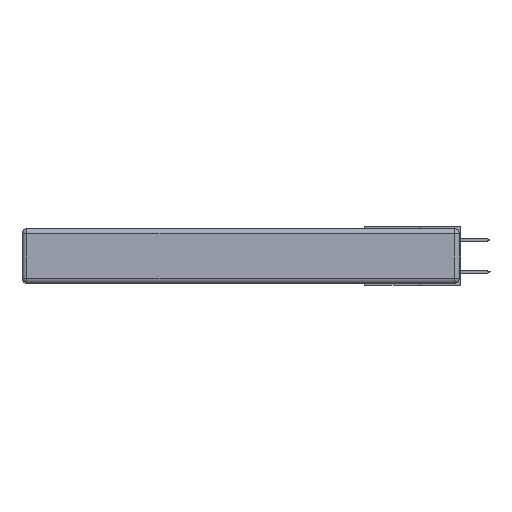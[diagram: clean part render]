
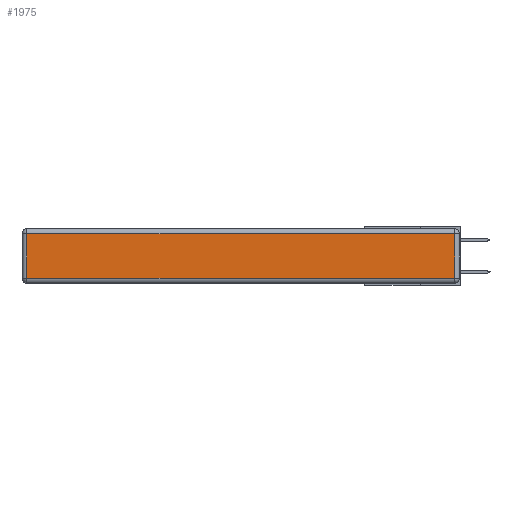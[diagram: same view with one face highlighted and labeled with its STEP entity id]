
A CAD part, left-side view. The second image highlights one B-rep face of the part: STEP entity #1975.
In plain terms, the highlighted planar face has unit normal (-1, 0, 0).
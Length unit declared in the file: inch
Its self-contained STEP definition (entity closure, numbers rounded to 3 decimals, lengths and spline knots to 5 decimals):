
#149 = LINE ( 'NONE', #11013, #15096 ) ;
#1152 = EDGE_CURVE ( 'NONE', #13067, #14570, #5375, .T. ) ;
#1941 = DIRECTION ( 'NONE',  ( 0., 0., -1. ) ) ;
#1975 = ADVANCED_FACE ( 'NONE', ( #10349 ), #14924, .T. ) ;
#2583 = VECTOR ( 'NONE', #1941, 39.37008 ) ;
#2803 = DIRECTION ( 'NONE',  ( 0., 0., 1. ) ) ;
#2914 = CARTESIAN_POINT ( 'NONE',  ( 0., 0.03, -0.03 ) ) ;
#4265 = ORIENTED_EDGE ( 'NONE', *, *, #11725, .T. ) ;
#4637 = VECTOR ( 'NONE', #11472, 39.37008 ) ;
#4708 = ORIENTED_EDGE ( 'NONE', *, *, #6170, .T. ) ;
#5375 = LINE ( 'NONE', #6583, #4637 ) ;
#5457 = EDGE_LOOP ( 'NONE', ( #12188, #4265, #4708, #12010 ) ) ;
#6170 = EDGE_CURVE ( 'NONE', #7872, #12443, #10819, .T. ) ;
#6190 = AXIS2_PLACEMENT_3D ( 'NONE', #7785, #9056, #9099 ) ;
#6583 = CARTESIAN_POINT ( 'NONE',  ( 0., 0., -0.313 ) ) ;
#7785 = CARTESIAN_POINT ( 'NONE',  ( 0., 0., -0.343 ) ) ;
#7872 = VERTEX_POINT ( 'NONE', #2914 ) ;
#7988 = DIRECTION ( 'NONE',  ( 0., 1., 0. ) ) ;
#8191 = VECTOR ( 'NONE', #7988, 39.37008 ) ;
#8332 = CARTESIAN_POINT ( 'NONE',  ( 0., 2.72, -0.313 ) ) ;
#9056 = DIRECTION ( 'NONE',  ( -1., 0., 0. ) ) ;
#9099 = DIRECTION ( 'NONE',  ( 0., 0., 1. ) ) ;
#10349 = FACE_OUTER_BOUND ( 'NONE', #5457, .T. ) ;
#10819 = LINE ( 'NONE', #11369, #8191 ) ;
#11013 = CARTESIAN_POINT ( 'NONE',  ( 0., 0.03, -0.343 ) ) ;
#11369 = CARTESIAN_POINT ( 'NONE',  ( 0., 2.75, -0.03 ) ) ;
#11404 = CARTESIAN_POINT ( 'NONE',  ( 0., 2.72, -0.343 ) ) ;
#11472 = DIRECTION ( 'NONE',  ( 0., -1., 0. ) ) ;
#11725 = EDGE_CURVE ( 'NONE', #14570, #7872, #149, .T. ) ;
#12010 = ORIENTED_EDGE ( 'NONE', *, *, #12426, .T. ) ;
#12188 = ORIENTED_EDGE ( 'NONE', *, *, #1152, .T. ) ;
#12426 = EDGE_CURVE ( 'NONE', #12443, #13067, #13570, .T. ) ;
#12443 = VERTEX_POINT ( 'NONE', #13808 ) ;
#13067 = VERTEX_POINT ( 'NONE', #8332 ) ;
#13175 = CARTESIAN_POINT ( 'NONE',  ( 0., 0.03, -0.313 ) ) ;
#13570 = LINE ( 'NONE', #11404, #2583 ) ;
#13808 = CARTESIAN_POINT ( 'NONE',  ( 0., 2.72, -0.03 ) ) ;
#14570 = VERTEX_POINT ( 'NONE', #13175 ) ;
#14924 = PLANE ( 'NONE',  #6190 ) ;
#15096 = VECTOR ( 'NONE', #2803, 39.37008 ) ;
